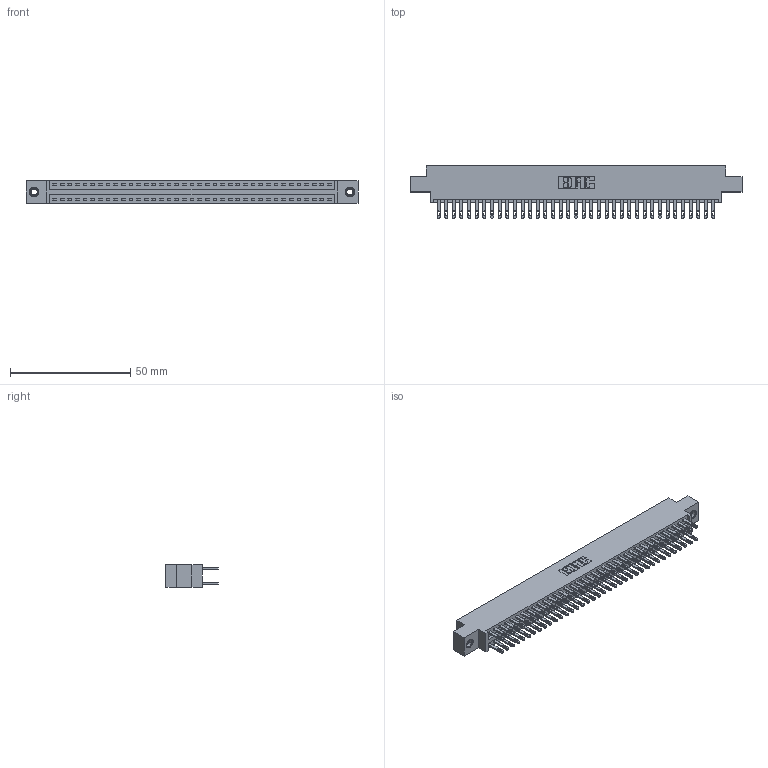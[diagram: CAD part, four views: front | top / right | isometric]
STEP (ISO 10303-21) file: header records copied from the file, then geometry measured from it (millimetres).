
FILE_DESCRIPTION (( 'STEP AP203' ), '1' );
FILE_NAME ('346-074-500-807.STEP', '2022-05-25T01:31:18', ( '' ), ( '' ), 'SwSTEP 2.0', 'SolidWorks 2020', '' );
FILE_SCHEMA (( 'CONFIG_CONTROL_DESIGN' ));
Length unit declared in the file: inch
Products named in the file (4): 345-292-001_345-293-100; 345-250-001_345-250-005-103; 346-074-500-807; 346 Part_0.170 Offset - 0.156 Dia-TI
Assembly tree (77 placements, depth 2):
  346-074-500-807
    346 Part_0.170 Offset - 0.156 Dia-TI
    345-292-001_345-293-100  x74
    345-250-001_345-250-005-103  x2
Bounding box: 138.05 x 21.84 x 9.4 mm (x, y, z)
Volume: 13480.7 mm3; surface area: 19439.4 mm2
Topology: 77 solids, 77 shells, 3738 faces, 11355 edges, 7562 vertices
Faces by surface type: plane 2258, cylinder 1464, cone 12, torus 4
Entity records: 26068 total; most frequent: CARTESIAN_POINT 4287, ORIENTED_EDGE 4214, DIRECTION 3857, EDGE_CURVE 2107, VECTOR 1803, LINE 1803, VERTEX_POINT 1400, AXIS2_PLACEMENT_3D 1027
